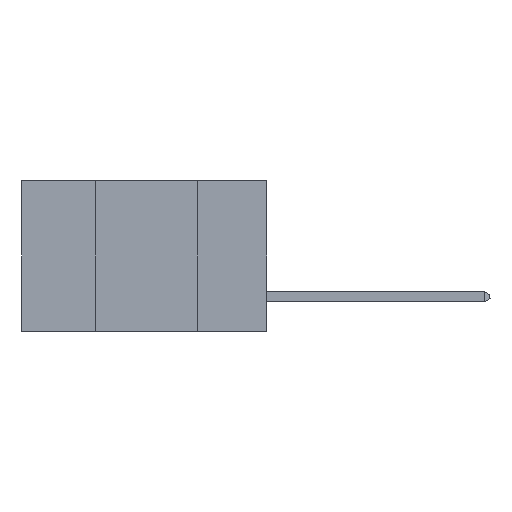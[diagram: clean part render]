
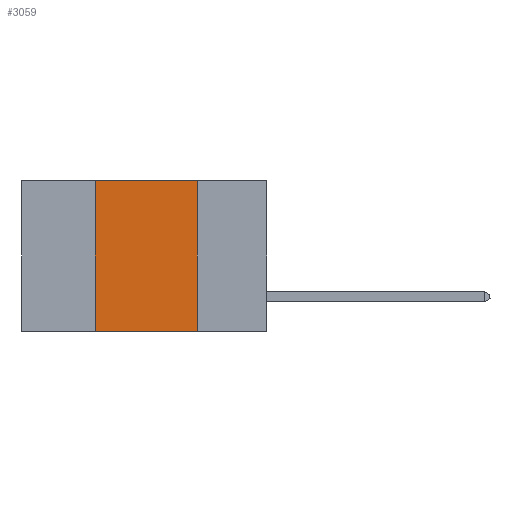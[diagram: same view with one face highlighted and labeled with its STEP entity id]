
A CAD part, left-side view. The second image highlights one B-rep face of the part: STEP entity #3059.
In plain terms, the highlighted planar face has unit normal (-1, 0, 0).
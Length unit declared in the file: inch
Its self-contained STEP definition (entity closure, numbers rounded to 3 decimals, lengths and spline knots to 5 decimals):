
#1962 = DIRECTION ( 'NONE',  ( 0., 0., -1. ) ) ;
#3059 = ADVANCED_FACE ( 'NONE', ( #26609 ), #7622, .F. ) ;
#3336 = DIRECTION ( 'NONE',  ( 0., -1., 0. ) ) ;
#5597 = DIRECTION ( 'NONE',  ( 0., 0., 1. ) ) ;
#6370 = VERTEX_POINT ( 'NONE', #26740 ) ;
#7258 = VECTOR ( 'NONE', #3336, 39.37008 ) ;
#7622 = PLANE ( 'NONE',  #14224 ) ;
#8239 = VERTEX_POINT ( 'NONE', #26340 ) ;
#9274 = VERTEX_POINT ( 'NONE', #12748 ) ;
#9880 = LINE ( 'NONE', #24537, #30496 ) ;
#10023 = CARTESIAN_POINT ( 'NONE',  ( 0., 0.42, 0. ) ) ;
#10839 = VECTOR ( 'NONE', #5597, 39.37008 ) ;
#11463 = ORIENTED_EDGE ( 'NONE', *, *, #16496, .F. ) ;
#12748 = CARTESIAN_POINT ( 'NONE',  ( 0., 0.17, -0.37 ) ) ;
#13474 = LINE ( 'NONE', #21976, #7258 ) ;
#13926 = VECTOR ( 'NONE', #1962, 39.37008 ) ;
#14224 = AXIS2_PLACEMENT_3D ( 'NONE', #23177, #31284, #28557 ) ;
#15419 = LINE ( 'NONE', #20647, #10839 ) ;
#16496 = EDGE_CURVE ( 'NONE', #6370, #9274, #33752, .T. ) ;
#17992 = CARTESIAN_POINT ( 'NONE',  ( 0., 0.17, 0. ) ) ;
#19424 = VERTEX_POINT ( 'NONE', #10023 ) ;
#19551 = EDGE_CURVE ( 'NONE', #8239, #9274, #13474, .T. ) ;
#20090 = ORIENTED_EDGE ( 'NONE', *, *, #31967, .F. ) ;
#20647 = CARTESIAN_POINT ( 'NONE',  ( 0., 0.42, 0. ) ) ;
#21196 = ORIENTED_EDGE ( 'NONE', *, *, #21836, .F. ) ;
#21836 = EDGE_CURVE ( 'NONE', #8239, #19424, #15419, .T. ) ;
#21976 = CARTESIAN_POINT ( 'NONE',  ( 0., 0.6, -0.37 ) ) ;
#23177 = CARTESIAN_POINT ( 'NONE',  ( 0., 0.6, 0. ) ) ;
#23505 = EDGE_LOOP ( 'NONE', ( #11463, #20090, #21196, #27375 ) ) ;
#24537 = CARTESIAN_POINT ( 'NONE',  ( 0., 0.6, 0. ) ) ;
#26340 = CARTESIAN_POINT ( 'NONE',  ( 0., 0.42, -0.37 ) ) ;
#26609 = FACE_OUTER_BOUND ( 'NONE', #23505, .T. ) ;
#26740 = CARTESIAN_POINT ( 'NONE',  ( 0., 0.17, 0. ) ) ;
#26796 = DIRECTION ( 'NONE',  ( 0., -1., 0. ) ) ;
#27375 = ORIENTED_EDGE ( 'NONE', *, *, #19551, .T. ) ;
#28557 = DIRECTION ( 'NONE',  ( 0., 0., -1. ) ) ;
#30496 = VECTOR ( 'NONE', #26796, 39.37008 ) ;
#31284 = DIRECTION ( 'NONE',  ( 1., 0., 0. ) ) ;
#31967 = EDGE_CURVE ( 'NONE', #19424, #6370, #9880, .T. ) ;
#33752 = LINE ( 'NONE', #17992, #13926 ) ;
